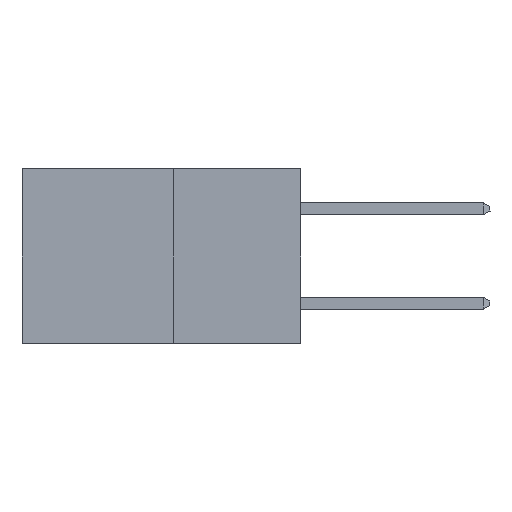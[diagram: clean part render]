
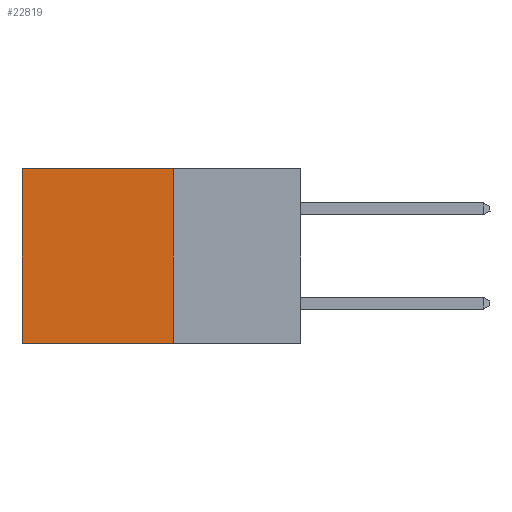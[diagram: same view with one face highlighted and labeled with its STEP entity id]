
A CAD part, left-side view. The second image highlights one B-rep face of the part: STEP entity #22819.
In plain terms, the highlighted planar face has unit normal (-1, 0, 0).
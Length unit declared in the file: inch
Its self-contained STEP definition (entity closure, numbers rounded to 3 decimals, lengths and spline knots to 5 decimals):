
#506 = CARTESIAN_POINT ( 'NONE',  ( 0.277, 0.27, 0. ) ) ;
#1023 = CARTESIAN_POINT ( 'NONE',  ( 0.277, 0.59, 0. ) ) ;
#1088 = LINE ( 'NONE', #18598, #14182 ) ;
#1901 = DIRECTION ( 'NONE',  ( 0., 0., -1. ) ) ;
#5135 = LINE ( 'NONE', #15755, #18108 ) ;
#7941 = EDGE_CURVE ( 'NONE', #9407, #16205, #1088, .T. ) ;
#9407 = VERTEX_POINT ( 'NONE', #1023 ) ;
#9488 = EDGE_CURVE ( 'NONE', #14097, #16205, #9882, .T. ) ;
#9608 = AXIS2_PLACEMENT_3D ( 'NONE', #10290, #15511, #33083 ) ;
#9882 = LINE ( 'NONE', #12000, #22739 ) ;
#10290 = CARTESIAN_POINT ( 'NONE',  ( 0.277, 0.27, -0.37 ) ) ;
#12000 = CARTESIAN_POINT ( 'NONE',  ( 0.277, 0.27, -0.37 ) ) ;
#12926 = PLANE ( 'NONE',  #9608 ) ;
#13045 = EDGE_CURVE ( 'NONE', #21620, #14097, #5135, .T. ) ;
#14097 = VERTEX_POINT ( 'NONE', #27693 ) ;
#14182 = VECTOR ( 'NONE', #1901, 39.37008 ) ;
#14525 = EDGE_CURVE ( 'NONE', #21620, #9407, #28727, .T. ) ;
#14936 = ORIENTED_EDGE ( 'NONE', *, *, #13045, .F. ) ;
#15511 = DIRECTION ( 'NONE',  ( 1., 0., 0. ) ) ;
#15618 = CARTESIAN_POINT ( 'NONE',  ( 0.277, 0.59, -0.37 ) ) ;
#15755 = CARTESIAN_POINT ( 'NONE',  ( 0.277, 0.27, -0.37 ) ) ;
#16205 = VERTEX_POINT ( 'NONE', #15618 ) ;
#16589 = CARTESIAN_POINT ( 'NONE',  ( 0.277, 0.27, 0. ) ) ;
#16754 = ORIENTED_EDGE ( 'NONE', *, *, #7941, .T. ) ;
#18108 = VECTOR ( 'NONE', #28393, 39.37008 ) ;
#18598 = CARTESIAN_POINT ( 'NONE',  ( 0.277, 0.59, -0.37 ) ) ;
#19525 = EDGE_LOOP ( 'NONE', ( #16754, #32254, #14936, #22129 ) ) ;
#20206 = FACE_OUTER_BOUND ( 'NONE', #19525, .T. ) ;
#21245 = VECTOR ( 'NONE', #29193, 39.37008 ) ;
#21620 = VERTEX_POINT ( 'NONE', #506 ) ;
#22129 = ORIENTED_EDGE ( 'NONE', *, *, #14525, .T. ) ;
#22739 = VECTOR ( 'NONE', #32221, 39.37008 ) ;
#22819 = ADVANCED_FACE ( 'NONE', ( #20206 ), #12926, .F. ) ;
#27693 = CARTESIAN_POINT ( 'NONE',  ( 0.277, 0.27, -0.37 ) ) ;
#28393 = DIRECTION ( 'NONE',  ( 0., 0., -1. ) ) ;
#28727 = LINE ( 'NONE', #16589, #21245 ) ;
#29193 = DIRECTION ( 'NONE',  ( 0., 1., 0. ) ) ;
#32221 = DIRECTION ( 'NONE',  ( 0., 1., 0. ) ) ;
#32254 = ORIENTED_EDGE ( 'NONE', *, *, #9488, .F. ) ;
#33083 = DIRECTION ( 'NONE',  ( 0., 0., -1. ) ) ;
